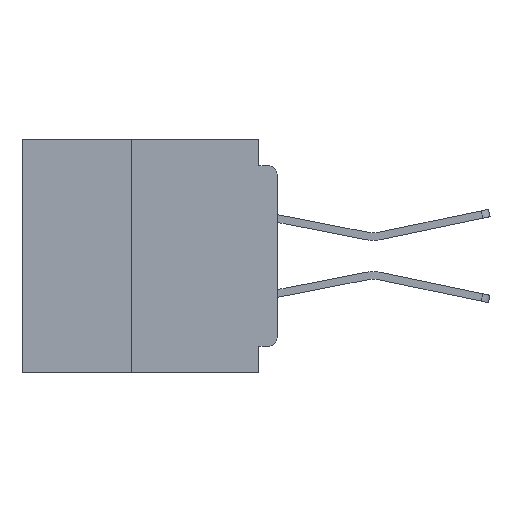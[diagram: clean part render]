
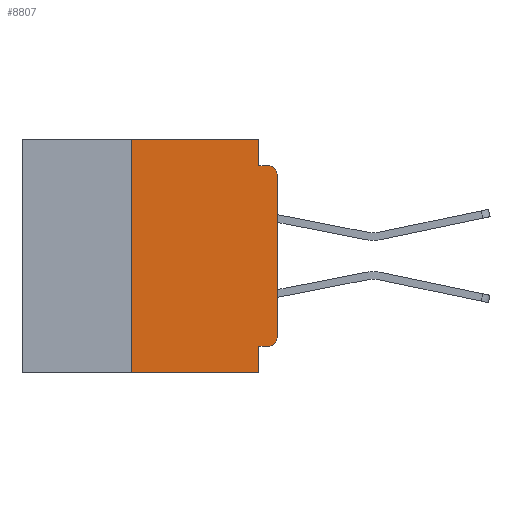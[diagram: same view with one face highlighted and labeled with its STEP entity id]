
A CAD part, left-side view. The second image highlights one B-rep face of the part: STEP entity #8807.
In plain terms, the highlighted planar face has unit normal (-1, 0, 0).
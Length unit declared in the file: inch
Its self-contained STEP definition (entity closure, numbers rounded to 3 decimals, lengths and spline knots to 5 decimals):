
#109 = CARTESIAN_POINT ( 'NONE',  ( 0., 0.031, -0.045 ) ) ;
#478 = CARTESIAN_POINT ( 'NONE',  ( 0., 0.031, 0. ) ) ;
#1184 = DIRECTION ( 'NONE',  ( 0., -1., 0. ) ) ;
#1931 = ORIENTED_EDGE ( 'NONE', *, *, #39021, .F. ) ;
#3062 = VERTEX_POINT ( 'NONE', #109 ) ;
#3169 = VERTEX_POINT ( 'NONE', #28089 ) ;
#3347 = ORIENTED_EDGE ( 'NONE', *, *, #19047, .F. ) ;
#3753 = VERTEX_POINT ( 'NONE', #29706 ) ;
#4322 = VERTEX_POINT ( 'NONE', #4727 ) ;
#4514 = EDGE_CURVE ( 'NONE', #32621, #7486, #12693, .T. ) ;
#4727 = CARTESIAN_POINT ( 'NONE',  ( 0., 0.25, -0.4 ) ) ;
#4974 = DIRECTION ( 'NONE',  ( 0., 0., 1. ) ) ;
#5758 = VECTOR ( 'NONE', #1184, 39.37008 ) ;
#6467 = VERTEX_POINT ( 'NONE', #39563 ) ;
#7336 = CARTESIAN_POINT ( 'NONE',  ( 0., 0., 0. ) ) ;
#7486 = VERTEX_POINT ( 'NONE', #478 ) ;
#8034 = CIRCLE ( 'NONE', #15820, 0.015 ) ;
#8172 = LINE ( 'NONE', #18992, #50462 ) ;
#8687 = LINE ( 'NONE', #7336, #30559 ) ;
#8807 = ADVANCED_FACE ( 'NONE', ( #23632 ), #45747, .F. ) ;
#9000 = DIRECTION ( 'NONE',  ( 0., 0., -1. ) ) ;
#9320 = CARTESIAN_POINT ( 'NONE',  ( 0., 0.437, -0.4 ) ) ;
#10885 = DIRECTION ( 'NONE',  ( 0., 0., -1. ) ) ;
#11016 = AXIS2_PLACEMENT_3D ( 'NONE', #29515, #33603, #9000 ) ;
#12693 = LINE ( 'NONE', #45110, #13973 ) ;
#13973 = VECTOR ( 'NONE', #44116, 39.37008 ) ;
#14232 = DIRECTION ( 'NONE',  ( -1., 0., 0. ) ) ;
#15820 = AXIS2_PLACEMENT_3D ( 'NONE', #18271, #46882, #22381 ) ;
#16014 = DIRECTION ( 'NONE',  ( 0., -1., 0. ) ) ;
#16133 = DIRECTION ( 'NONE',  ( 0., 1., 0. ) ) ;
#17788 = CARTESIAN_POINT ( 'NONE',  ( 0., 0.015, -0.355 ) ) ;
#18261 = EDGE_CURVE ( 'NONE', #3753, #6467, #8034, .T. ) ;
#18271 = CARTESIAN_POINT ( 'NONE',  ( 0., 0.015, -0.06 ) ) ;
#18729 = LINE ( 'NONE', #52839, #40520 ) ;
#18890 = LINE ( 'NONE', #43965, #39406 ) ;
#18992 = CARTESIAN_POINT ( 'NONE',  ( 0., 0.031, 0. ) ) ;
#19047 = EDGE_CURVE ( 'NONE', #38924, #49054, #18890, .T. ) ;
#19451 = VERTEX_POINT ( 'NONE', #17788 ) ;
#21142 = EDGE_LOOP ( 'NONE', ( #41124, #42781, #35967, #49101, #32238, #46469, #48592, #3347, #1931, #29052 ) ) ;
#21776 = EDGE_CURVE ( 'NONE', #4322, #49054, #28966, .T. ) ;
#22381 = DIRECTION ( 'NONE',  ( 0., 0., -1. ) ) ;
#22906 = AXIS2_PLACEMENT_3D ( 'NONE', #38789, #14232, #42884 ) ;
#23307 = VECTOR ( 'NONE', #4974, 39.37008 ) ;
#23632 = FACE_OUTER_BOUND ( 'NONE', #21142, .T. ) ;
#23687 = CARTESIAN_POINT ( 'NONE',  ( 0., 0.031, -0.355 ) ) ;
#24071 = EDGE_CURVE ( 'NONE', #19451, #3169, #40811, .T. ) ;
#24273 = EDGE_CURVE ( 'NONE', #3169, #3753, #8687, .T. ) ;
#24584 = CARTESIAN_POINT ( 'NONE',  ( 0., 0.25, 0. ) ) ;
#26957 = CARTESIAN_POINT ( 'NONE',  ( 0., 0.031, -0.4 ) ) ;
#28089 = CARTESIAN_POINT ( 'NONE',  ( 0., 0., -0.34 ) ) ;
#28966 = LINE ( 'NONE', #9320, #5758 ) ;
#29052 = ORIENTED_EDGE ( 'NONE', *, *, #24071, .T. ) ;
#29515 = CARTESIAN_POINT ( 'NONE',  ( 0., 0.437, 0. ) ) ;
#29706 = CARTESIAN_POINT ( 'NONE',  ( 0., 0., -0.06 ) ) ;
#30559 = VECTOR ( 'NONE', #36092, 39.37008 ) ;
#32238 = ORIENTED_EDGE ( 'NONE', *, *, #4514, .F. ) ;
#32621 = VERTEX_POINT ( 'NONE', #24584 ) ;
#32792 = EDGE_CURVE ( 'NONE', #4322, #32621, #46342, .T. ) ;
#33603 = DIRECTION ( 'NONE',  ( 1., 0., 0. ) ) ;
#35967 = ORIENTED_EDGE ( 'NONE', *, *, #50813, .F. ) ;
#36092 = DIRECTION ( 'NONE',  ( 0., 0., 1. ) ) ;
#36599 = CARTESIAN_POINT ( 'NONE',  ( 0., 0., -0.355 ) ) ;
#38789 = CARTESIAN_POINT ( 'NONE',  ( 0., 0.015, -0.34 ) ) ;
#38924 = VERTEX_POINT ( 'NONE', #23687 ) ;
#39021 = EDGE_CURVE ( 'NONE', #19451, #38924, #51386, .T. ) ;
#39406 = VECTOR ( 'NONE', #48053, 39.37008 ) ;
#39563 = CARTESIAN_POINT ( 'NONE',  ( 0., 0.015, -0.045 ) ) ;
#40520 = VECTOR ( 'NONE', #16014, 39.37008 ) ;
#40811 = CIRCLE ( 'NONE', #22906, 0.015 ) ;
#41124 = ORIENTED_EDGE ( 'NONE', *, *, #24273, .T. ) ;
#42146 = CARTESIAN_POINT ( 'NONE',  ( 0., 0.25, -0.4 ) ) ;
#42781 = ORIENTED_EDGE ( 'NONE', *, *, #18261, .T. ) ;
#42884 = DIRECTION ( 'NONE',  ( 0., 0., -1. ) ) ;
#43965 = CARTESIAN_POINT ( 'NONE',  ( 0., 0.031, -0.4 ) ) ;
#44116 = DIRECTION ( 'NONE',  ( 0., -1., 0. ) ) ;
#45110 = CARTESIAN_POINT ( 'NONE',  ( 0., 0.437, 0. ) ) ;
#45747 = PLANE ( 'NONE',  #11016 ) ;
#46342 = LINE ( 'NONE', #42146, #23307 ) ;
#46469 = ORIENTED_EDGE ( 'NONE', *, *, #32792, .F. ) ;
#46478 = EDGE_CURVE ( 'NONE', #7486, #3062, #8172, .T. ) ;
#46882 = DIRECTION ( 'NONE',  ( -1., 0., 0. ) ) ;
#48053 = DIRECTION ( 'NONE',  ( 0., 0., -1. ) ) ;
#48592 = ORIENTED_EDGE ( 'NONE', *, *, #21776, .T. ) ;
#49054 = VERTEX_POINT ( 'NONE', #26957 ) ;
#49101 = ORIENTED_EDGE ( 'NONE', *, *, #46478, .F. ) ;
#50117 = VECTOR ( 'NONE', #16133, 39.37008 ) ;
#50462 = VECTOR ( 'NONE', #10885, 39.37008 ) ;
#50813 = EDGE_CURVE ( 'NONE', #3062, #6467, #18729, .T. ) ;
#51386 = LINE ( 'NONE', #36599, #50117 ) ;
#52839 = CARTESIAN_POINT ( 'NONE',  ( 0., 0., -0.045 ) ) ;
